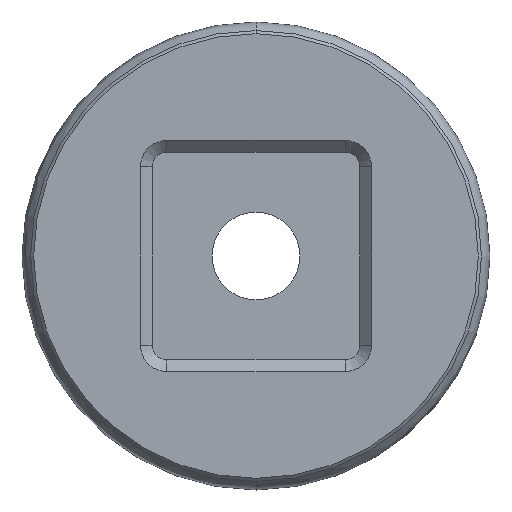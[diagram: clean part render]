
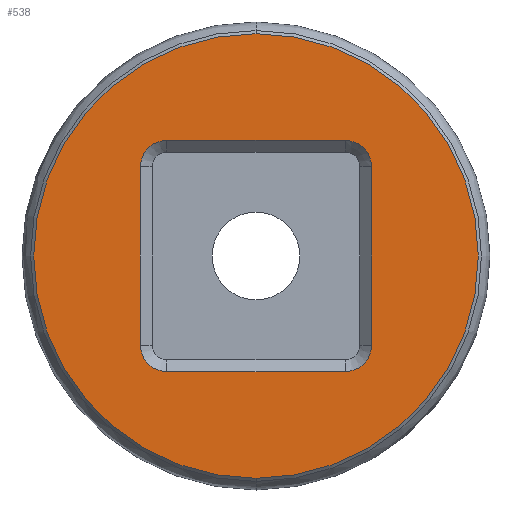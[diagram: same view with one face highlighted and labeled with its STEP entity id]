
A CAD part, front view. The second image highlights one B-rep face of the part: STEP entity #538.
In plain terms, the highlighted planar face has unit normal (0, -1, 0).
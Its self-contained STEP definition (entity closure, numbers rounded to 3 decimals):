
#6 = DIRECTION ( 'NONE',  ( 0., 1., 0. ) ) ;
#8 = VERTEX_POINT ( 'NONE', #502 ) ;
#24 = CIRCLE ( 'NONE', #396, 0.9 ) ;
#33 = CARTESIAN_POINT ( 'NONE',  ( -210.948, 58.134, -2.05 ) ) ;
#38 = VECTOR ( 'NONE', #303, 1000. ) ;
#47 = ORIENTED_EDGE ( 'NONE', *, *, #371, .T. ) ;
#51 = AXIS2_PLACEMENT_3D ( 'NONE', #779, #132, #584 ) ;
#62 = EDGE_CURVE ( 'NONE', #253, #550, #645, .T. ) ;
#67 = CARTESIAN_POINT ( 'NONE',  ( -203.048, 58.134, -2.05 ) ) ;
#76 = CARTESIAN_POINT ( 'NONE',  ( -210.048, 58.134, 4.95 ) ) ;
#90 = DIRECTION ( 'NONE',  ( 0., 0., -1. ) ) ;
#97 = EDGE_LOOP ( 'NONE', ( #202, #683 ) ) ;
#101 = DIRECTION ( 'NONE',  ( 0., 0., 1. ) ) ;
#126 = LINE ( 'NONE', #765, #906 ) ;
#132 = DIRECTION ( 'NONE',  ( 0., 1., 0. ) ) ;
#140 = CARTESIAN_POINT ( 'NONE',  ( -203.948, 58.134, -2.05 ) ) ;
#143 = CARTESIAN_POINT ( 'NONE',  ( -206.998, 58.134, 1. ) ) ;
#185 = AXIS2_PLACEMENT_3D ( 'NONE', #741, #312, #662 ) ;
#202 = ORIENTED_EDGE ( 'NONE', *, *, #439, .F. ) ;
#224 = DIRECTION ( 'NONE',  ( 0., 1., 0. ) ) ;
#225 = CARTESIAN_POINT ( 'NONE',  ( -210.948, 58.134, 1. ) ) ;
#233 = AXIS2_PLACEMENT_3D ( 'NONE', #856, #224, #444 ) ;
#243 = FACE_BOUND ( 'NONE', #305, .T. ) ;
#249 = VECTOR ( 'NONE', #101, 1000. ) ;
#253 = VERTEX_POINT ( 'NONE', #272 ) ;
#256 = ORIENTED_EDGE ( 'NONE', *, *, #316, .T. ) ;
#272 = CARTESIAN_POINT ( 'NONE',  ( -203.948, 58.134, 4.95 ) ) ;
#286 = CARTESIAN_POINT ( 'NONE',  ( -206.998, 58.134, -6.6 ) ) ;
#289 = ORIENTED_EDGE ( 'NONE', *, *, #736, .T. ) ;
#291 = CARTESIAN_POINT ( 'NONE',  ( -210.948, 58.134, 4.05 ) ) ;
#296 = DIRECTION ( 'NONE',  ( 0., 0., -1. ) ) ;
#298 = LINE ( 'NONE', #637, #38 ) ;
#300 = ORIENTED_EDGE ( 'NONE', *, *, #862, .T. ) ;
#303 = DIRECTION ( 'NONE',  ( 1., 0., 0. ) ) ;
#305 = EDGE_LOOP ( 'NONE', ( #688, #300, #47, #705, #738, #256, #832, #289 ) ) ;
#312 = DIRECTION ( 'NONE',  ( 0., 1., 0. ) ) ;
#316 = EDGE_CURVE ( 'NONE', #802, #8, #440, .T. ) ;
#343 = VERTEX_POINT ( 'NONE', #76 ) ;
#371 = EDGE_CURVE ( 'NONE', #343, #253, #298, .T. ) ;
#396 = AXIS2_PLACEMENT_3D ( 'NONE', #755, #844, #296 ) ;
#397 = PLANE ( 'NONE',  #594 ) ;
#415 = DIRECTION ( 'NONE',  ( -1., 0., 0. ) ) ;
#439 = EDGE_CURVE ( 'NONE', #483, #761, #471, .T. ) ;
#440 = CIRCLE ( 'NONE', #873, 0.9 ) ;
#444 = DIRECTION ( 'NONE',  ( 0., 0., -1. ) ) ;
#446 = DIRECTION ( 'NONE',  ( 0., 1., 0. ) ) ;
#462 = DIRECTION ( 'NONE',  ( 0., -1., 0. ) ) ;
#471 = CIRCLE ( 'NONE', #499, 7.6 ) ;
#480 = EDGE_CURVE ( 'NONE', #627, #837, #864, .T. ) ;
#483 = VERTEX_POINT ( 'NONE', #816 ) ;
#495 = LINE ( 'NONE', #773, #663 ) ;
#499 = AXIS2_PLACEMENT_3D ( 'NONE', #143, #446, #721 ) ;
#502 = CARTESIAN_POINT ( 'NONE',  ( -203.948, 58.134, -2.95 ) ) ;
#538 = ADVANCED_FACE ( 'NONE', ( #724, #243 ), #397, .T. ) ;
#550 = VERTEX_POINT ( 'NONE', #597 ) ;
#584 = DIRECTION ( 'NONE',  ( 0., 0., 1. ) ) ;
#594 = AXIS2_PLACEMENT_3D ( 'NONE', #600, #462, #90 ) ;
#597 = CARTESIAN_POINT ( 'NONE',  ( -203.048, 58.134, 4.05 ) ) ;
#600 = CARTESIAN_POINT ( 'NONE',  ( -206.998, 58.134, 1. ) ) ;
#627 = VERTEX_POINT ( 'NONE', #33 ) ;
#637 = CARTESIAN_POINT ( 'NONE',  ( -206.998, 58.134, 4.95 ) ) ;
#645 = CIRCLE ( 'NONE', #185, 0.9 ) ;
#662 = DIRECTION ( 'NONE',  ( 0., 0., -1. ) ) ;
#663 = VECTOR ( 'NONE', #789, 1000. ) ;
#681 = EDGE_CURVE ( 'NONE', #8, #917, #126, .T. ) ;
#683 = ORIENTED_EDGE ( 'NONE', *, *, #750, .F. ) ;
#688 = ORIENTED_EDGE ( 'NONE', *, *, #480, .T. ) ;
#705 = ORIENTED_EDGE ( 'NONE', *, *, #62, .T. ) ;
#709 = DIRECTION ( 'NONE',  ( 0., 0., -1. ) ) ;
#721 = DIRECTION ( 'NONE',  ( 0., 0., 1. ) ) ;
#724 = FACE_OUTER_BOUND ( 'NONE', #97, .T. ) ;
#736 = EDGE_CURVE ( 'NONE', #917, #627, #24, .T. ) ;
#738 = ORIENTED_EDGE ( 'NONE', *, *, #777, .T. ) ;
#741 = CARTESIAN_POINT ( 'NONE',  ( -203.948, 58.134, 4.05 ) ) ;
#750 = EDGE_CURVE ( 'NONE', #761, #483, #919, .T. ) ;
#755 = CARTESIAN_POINT ( 'NONE',  ( -210.048, 58.134, -2.05 ) ) ;
#761 = VERTEX_POINT ( 'NONE', #286 ) ;
#765 = CARTESIAN_POINT ( 'NONE',  ( -206.998, 58.134, -2.95 ) ) ;
#773 = CARTESIAN_POINT ( 'NONE',  ( -203.048, 58.134, 1. ) ) ;
#777 = EDGE_CURVE ( 'NONE', #550, #802, #495, .T. ) ;
#779 = CARTESIAN_POINT ( 'NONE',  ( -206.998, 58.134, 1. ) ) ;
#780 = CIRCLE ( 'NONE', #233, 0.9 ) ;
#789 = DIRECTION ( 'NONE',  ( 0., 0., -1. ) ) ;
#802 = VERTEX_POINT ( 'NONE', #67 ) ;
#816 = CARTESIAN_POINT ( 'NONE',  ( -206.998, 58.134, 8.6 ) ) ;
#832 = ORIENTED_EDGE ( 'NONE', *, *, #681, .T. ) ;
#837 = VERTEX_POINT ( 'NONE', #291 ) ;
#844 = DIRECTION ( 'NONE',  ( 0., 1., 0. ) ) ;
#856 = CARTESIAN_POINT ( 'NONE',  ( -210.048, 58.134, 4.05 ) ) ;
#862 = EDGE_CURVE ( 'NONE', #837, #343, #780, .T. ) ;
#864 = LINE ( 'NONE', #225, #249 ) ;
#872 = CARTESIAN_POINT ( 'NONE',  ( -210.048, 58.134, -2.95 ) ) ;
#873 = AXIS2_PLACEMENT_3D ( 'NONE', #140, #6, #709 ) ;
#906 = VECTOR ( 'NONE', #415, 1000. ) ;
#917 = VERTEX_POINT ( 'NONE', #872 ) ;
#919 = CIRCLE ( 'NONE', #51, 7.6 ) ;
